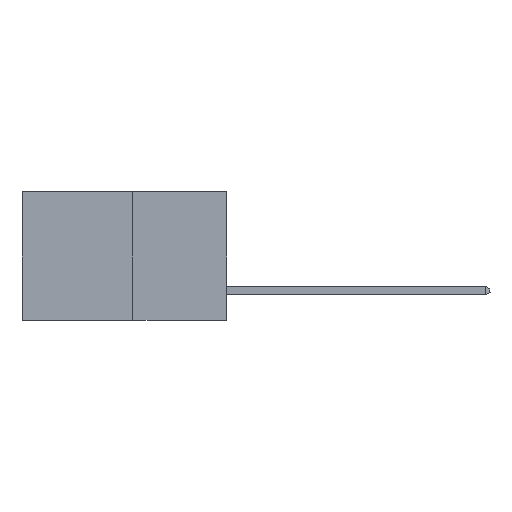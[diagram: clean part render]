
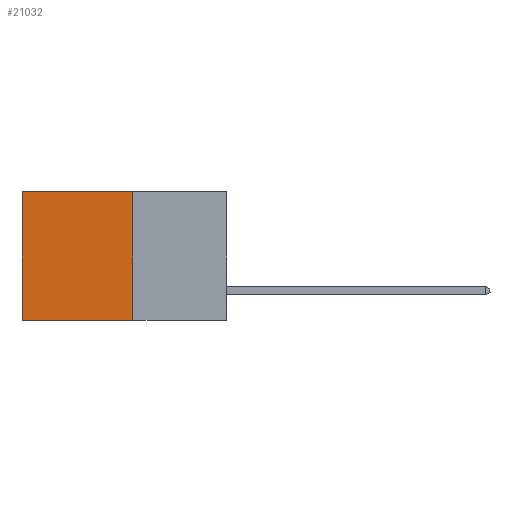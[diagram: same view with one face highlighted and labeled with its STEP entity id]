
A CAD part, left-side view. The second image highlights one B-rep face of the part: STEP entity #21032.
In plain terms, the highlighted planar face has unit normal (-1, 0, 0).
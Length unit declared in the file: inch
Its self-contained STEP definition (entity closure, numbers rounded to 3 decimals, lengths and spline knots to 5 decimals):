
#815 = EDGE_LOOP ( 'NONE', ( #15222, #1602, #16561, #10709 ) ) ;
#1602 = ORIENTED_EDGE ( 'NONE', *, *, #19300, .F. ) ;
#1814 = VERTEX_POINT ( 'NONE', #21091 ) ;
#2343 = LINE ( 'NONE', #17551, #16557 ) ;
#2818 = CARTESIAN_POINT ( 'NONE',  ( 0.277, 0.59, -0.37 ) ) ;
#3811 = CARTESIAN_POINT ( 'NONE',  ( 0.277, 0.59, -0.37 ) ) ;
#4855 = VECTOR ( 'NONE', #11501, 39.37008 ) ;
#4994 = AXIS2_PLACEMENT_3D ( 'NONE', #18670, #7139, #20572 ) ;
#6906 = EDGE_CURVE ( 'NONE', #17339, #21560, #15731, .T. ) ;
#7139 = DIRECTION ( 'NONE',  ( 1., 0., 0. ) ) ;
#7724 = VERTEX_POINT ( 'NONE', #15660 ) ;
#8095 = VECTOR ( 'NONE', #20899, 39.37008 ) ;
#8375 = EDGE_CURVE ( 'NONE', #1814, #7724, #2343, .T. ) ;
#8717 = LINE ( 'NONE', #19010, #8095 ) ;
#10709 = ORIENTED_EDGE ( 'NONE', *, *, #23907, .T. ) ;
#11501 = DIRECTION ( 'NONE',  ( 0., 0., -1. ) ) ;
#11962 = FACE_OUTER_BOUND ( 'NONE', #815, .T. ) ;
#12611 = CARTESIAN_POINT ( 'NONE',  ( 0.277, 0.27, 0. ) ) ;
#12990 = LINE ( 'NONE', #12611, #23113 ) ;
#15222 = ORIENTED_EDGE ( 'NONE', *, *, #6906, .T. ) ;
#15660 = CARTESIAN_POINT ( 'NONE',  ( 0.277, 0.27, -0.37 ) ) ;
#15731 = LINE ( 'NONE', #3811, #4855 ) ;
#16557 = VECTOR ( 'NONE', #19450, 39.37008 ) ;
#16561 = ORIENTED_EDGE ( 'NONE', *, *, #8375, .F. ) ;
#16731 = CARTESIAN_POINT ( 'NONE',  ( 0.277, 0.59, 0. ) ) ;
#17339 = VERTEX_POINT ( 'NONE', #16731 ) ;
#17551 = CARTESIAN_POINT ( 'NONE',  ( 0.277, 0.27, -0.37 ) ) ;
#18670 = CARTESIAN_POINT ( 'NONE',  ( 0.277, 0.27, -0.37 ) ) ;
#19010 = CARTESIAN_POINT ( 'NONE',  ( 0.277, 0.27, -0.37 ) ) ;
#19300 = EDGE_CURVE ( 'NONE', #7724, #21560, #8717, .T. ) ;
#19450 = DIRECTION ( 'NONE',  ( 0., 0., -1. ) ) ;
#20572 = DIRECTION ( 'NONE',  ( 0., 0., -1. ) ) ;
#20899 = DIRECTION ( 'NONE',  ( 0., 1., 0. ) ) ;
#21032 = ADVANCED_FACE ( 'NONE', ( #11962 ), #24277, .F. ) ;
#21091 = CARTESIAN_POINT ( 'NONE',  ( 0.277, 0.27, 0. ) ) ;
#21560 = VERTEX_POINT ( 'NONE', #2818 ) ;
#22085 = DIRECTION ( 'NONE',  ( 0., 1., 0. ) ) ;
#23113 = VECTOR ( 'NONE', #22085, 39.37008 ) ;
#23907 = EDGE_CURVE ( 'NONE', #1814, #17339, #12990, .T. ) ;
#24277 = PLANE ( 'NONE',  #4994 ) ;
